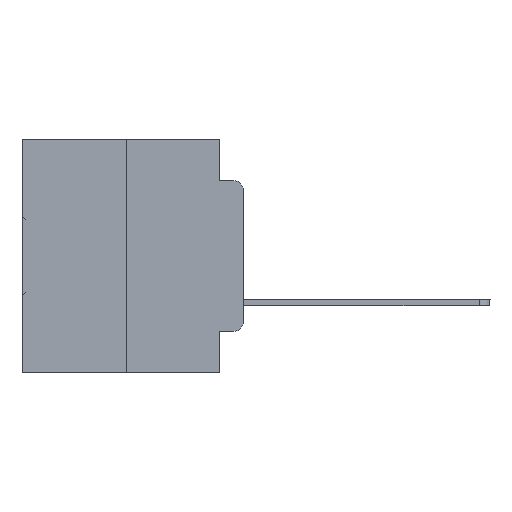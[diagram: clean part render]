
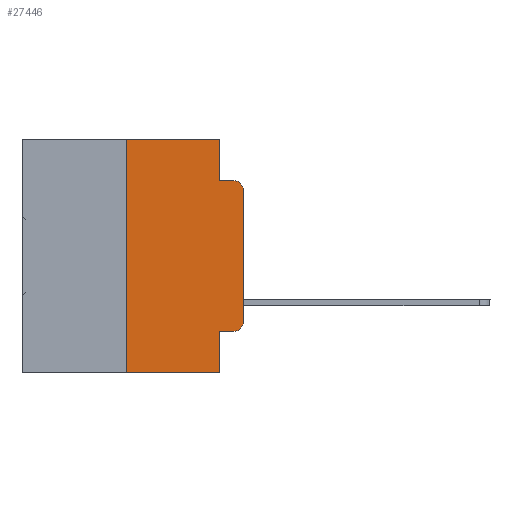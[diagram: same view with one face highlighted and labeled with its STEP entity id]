
A CAD part, left-side view. The second image highlights one B-rep face of the part: STEP entity #27446.
In plain terms, the highlighted planar face has unit normal (-1, 0, 0).
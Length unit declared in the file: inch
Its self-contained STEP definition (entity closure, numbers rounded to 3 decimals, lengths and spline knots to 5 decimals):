
#28 = CARTESIAN_POINT ( 'NONE',  ( 0., 0.25, -0.5 ) ) ;
#305 = LINE ( 'NONE', #20989, #16869 ) ;
#550 = EDGE_CURVE ( 'NONE', #8710, #26644, #30867, .T. ) ;
#878 = DIRECTION ( 'NONE',  ( 0., -1., 0. ) ) ;
#1096 = EDGE_CURVE ( 'NONE', #6689, #25960, #21707, .T. ) ;
#1161 = ORIENTED_EDGE ( 'NONE', *, *, #26203, .F. ) ;
#1264 = DIRECTION ( 'NONE',  ( 1., 0., 0. ) ) ;
#2345 = DIRECTION ( 'NONE',  ( 0., 0., 1. ) ) ;
#3045 = ORIENTED_EDGE ( 'NONE', *, *, #3897, .F. ) ;
#3364 = CARTESIAN_POINT ( 'NONE',  ( 0., 0.051, -0.5 ) ) ;
#3475 = DIRECTION ( 'NONE',  ( 0., 0., -1. ) ) ;
#3897 = EDGE_CURVE ( 'NONE', #8055, #32612, #5760, .T. ) ;
#5483 = CARTESIAN_POINT ( 'NONE',  ( 0., 0.25, 0. ) ) ;
#5594 = DIRECTION ( 'NONE',  ( 0., 0., -1. ) ) ;
#5760 = LINE ( 'NONE', #11189, #8577 ) ;
#5998 = AXIS2_PLACEMENT_3D ( 'NONE', #28660, #13625, #10739 ) ;
#6201 = CARTESIAN_POINT ( 'NONE',  ( 0., 0.051, -0.0885 ) ) ;
#6459 = VERTEX_POINT ( 'NONE', #24641 ) ;
#6594 = CARTESIAN_POINT ( 'NONE',  ( 0., 0.051, -0.0885 ) ) ;
#6689 = VERTEX_POINT ( 'NONE', #28 ) ;
#7116 = VECTOR ( 'NONE', #31852, 39.37008 ) ;
#7631 = LINE ( 'NONE', #25894, #28944 ) ;
#8055 = VERTEX_POINT ( 'NONE', #14290 ) ;
#8250 = CARTESIAN_POINT ( 'NONE',  ( 0., 0.051, 0. ) ) ;
#8562 = AXIS2_PLACEMENT_3D ( 'NONE', #15829, #13300, #17686 ) ;
#8577 = VECTOR ( 'NONE', #5594, 39.37008 ) ;
#8710 = VERTEX_POINT ( 'NONE', #23362 ) ;
#10059 = VECTOR ( 'NONE', #3475, 39.37008 ) ;
#10739 = DIRECTION ( 'NONE',  ( 0., 0., -1. ) ) ;
#11189 = CARTESIAN_POINT ( 'NONE',  ( 0., 0.051, 0. ) ) ;
#11463 = FACE_OUTER_BOUND ( 'NONE', #18891, .T. ) ;
#12163 = ORIENTED_EDGE ( 'NONE', *, *, #13878, .F. ) ;
#13300 = DIRECTION ( 'NONE',  ( -1., 0., 0. ) ) ;
#13508 = CARTESIAN_POINT ( 'NONE',  ( 0., 0.02, -0.0885 ) ) ;
#13619 = EDGE_CURVE ( 'NONE', #25960, #8055, #31893, .T. ) ;
#13625 = DIRECTION ( 'NONE',  ( -1., 0., 0. ) ) ;
#13878 = EDGE_CURVE ( 'NONE', #32612, #17048, #31443, .T. ) ;
#14290 = CARTESIAN_POINT ( 'NONE',  ( 0., 0.051, 0. ) ) ;
#15829 = CARTESIAN_POINT ( 'NONE',  ( 0., 0.02, -0.1085 ) ) ;
#16017 = DIRECTION ( 'NONE',  ( 0., 0., -1. ) ) ;
#16188 = PLANE ( 'NONE',  #23106 ) ;
#16416 = EDGE_CURVE ( 'NONE', #26644, #6459, #7631, .T. ) ;
#16501 = EDGE_CURVE ( 'NONE', #20271, #8710, #23862, .T. ) ;
#16534 = DIRECTION ( 'NONE',  ( 0., -1., 0. ) ) ;
#16869 = VECTOR ( 'NONE', #31315, 39.37008 ) ;
#17048 = VERTEX_POINT ( 'NONE', #13508 ) ;
#17686 = DIRECTION ( 'NONE',  ( 0., 0., -1. ) ) ;
#17960 = ORIENTED_EDGE ( 'NONE', *, *, #16501, .T. ) ;
#18513 = CARTESIAN_POINT ( 'NONE',  ( 0., 0., -0.3915 ) ) ;
#18891 = EDGE_LOOP ( 'NONE', ( #28121, #19306, #12163, #3045, #19900, #29421, #21693, #1161, #17960, #32849 ) ) ;
#19025 = EDGE_CURVE ( 'NONE', #6459, #17048, #33412, .T. ) ;
#19306 = ORIENTED_EDGE ( 'NONE', *, *, #19025, .T. ) ;
#19900 = ORIENTED_EDGE ( 'NONE', *, *, #13619, .F. ) ;
#20271 = VERTEX_POINT ( 'NONE', #25180 ) ;
#20989 = CARTESIAN_POINT ( 'NONE',  ( 0., 0.473, -0.5 ) ) ;
#21505 = CARTESIAN_POINT ( 'NONE',  ( 0., 0.051, -0.4115 ) ) ;
#21693 = ORIENTED_EDGE ( 'NONE', *, *, #24185, .T. ) ;
#21707 = LINE ( 'NONE', #26757, #7116 ) ;
#21795 = CARTESIAN_POINT ( 'NONE',  ( 0., 0.473, 0. ) ) ;
#23106 = AXIS2_PLACEMENT_3D ( 'NONE', #21795, #1264, #16017 ) ;
#23362 = CARTESIAN_POINT ( 'NONE',  ( 0., 0.02, -0.4115 ) ) ;
#23695 = DIRECTION ( 'NONE',  ( 0., -1., 0. ) ) ;
#23862 = LINE ( 'NONE', #21505, #26766 ) ;
#24185 = EDGE_CURVE ( 'NONE', #6689, #25496, #305, .T. ) ;
#24440 = CARTESIAN_POINT ( 'NONE',  ( 0., 0.473, 0. ) ) ;
#24641 = CARTESIAN_POINT ( 'NONE',  ( 0., 0., -0.1085 ) ) ;
#25141 = VECTOR ( 'NONE', #16534, 39.37008 ) ;
#25180 = CARTESIAN_POINT ( 'NONE',  ( 0., 0.051, -0.4115 ) ) ;
#25496 = VERTEX_POINT ( 'NONE', #3364 ) ;
#25894 = CARTESIAN_POINT ( 'NONE',  ( 0., 0., 0. ) ) ;
#25960 = VERTEX_POINT ( 'NONE', #5483 ) ;
#26203 = EDGE_CURVE ( 'NONE', #20271, #25496, #31438, .T. ) ;
#26644 = VERTEX_POINT ( 'NONE', #18513 ) ;
#26757 = CARTESIAN_POINT ( 'NONE',  ( 0., 0.25, 0. ) ) ;
#26766 = VECTOR ( 'NONE', #23695, 39.37008 ) ;
#27446 = ADVANCED_FACE ( 'NONE', ( #11463 ), #16188, .F. ) ;
#28121 = ORIENTED_EDGE ( 'NONE', *, *, #16416, .T. ) ;
#28660 = CARTESIAN_POINT ( 'NONE',  ( 0., 0.02, -0.3915 ) ) ;
#28942 = VECTOR ( 'NONE', #878, 39.37008 ) ;
#28944 = VECTOR ( 'NONE', #2345, 39.37008 ) ;
#29421 = ORIENTED_EDGE ( 'NONE', *, *, #1096, .F. ) ;
#30867 = CIRCLE ( 'NONE', #5998, 0.02 ) ;
#31315 = DIRECTION ( 'NONE',  ( 0., -1., 0. ) ) ;
#31438 = LINE ( 'NONE', #8250, #10059 ) ;
#31443 = LINE ( 'NONE', #6201, #25141 ) ;
#31852 = DIRECTION ( 'NONE',  ( 0., 0., 1. ) ) ;
#31893 = LINE ( 'NONE', #24440, #28942 ) ;
#32612 = VERTEX_POINT ( 'NONE', #6594 ) ;
#32849 = ORIENTED_EDGE ( 'NONE', *, *, #550, .T. ) ;
#33412 = CIRCLE ( 'NONE', #8562, 0.02 ) ;
